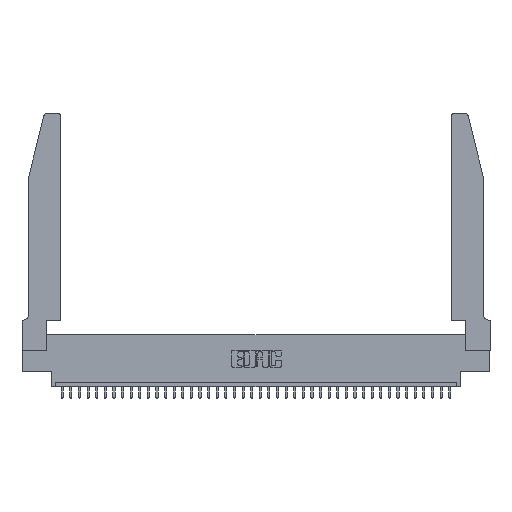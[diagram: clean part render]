
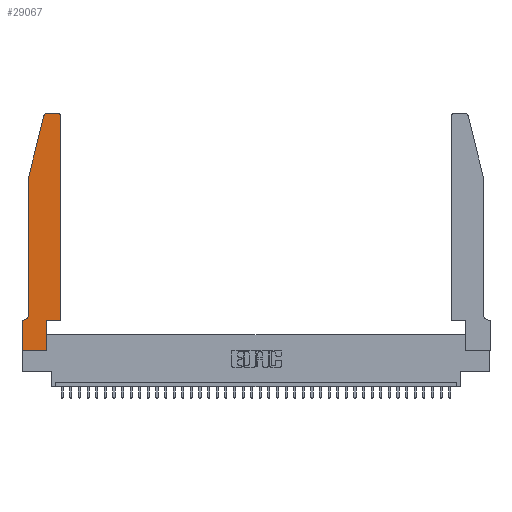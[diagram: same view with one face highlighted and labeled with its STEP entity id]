
A CAD part, top view. The second image highlights one B-rep face of the part: STEP entity #29067.
In plain terms, the highlighted planar face has unit normal (0, 0, 1).
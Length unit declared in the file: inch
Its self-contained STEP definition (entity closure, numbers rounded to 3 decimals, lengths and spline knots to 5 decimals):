
#1002 = CARTESIAN_POINT ( 'NONE',  ( 0.4505, 0.35, 0.37 ) ) ;
#1576 = VECTOR ( 'NONE', #4024, 39.37008 ) ;
#1795 = VECTOR ( 'NONE', #8593, 39.37008 ) ;
#1898 = CARTESIAN_POINT ( 'NONE',  ( 0.4205, 2.75, 0.37 ) ) ;
#2203 = VERTEX_POINT ( 'NONE', #10941 ) ;
#2248 = CARTESIAN_POINT ( 'NONE',  ( 0.25487, 2.72718, 0.37 ) ) ;
#2390 = LINE ( 'NONE', #22904, #25029 ) ;
#2543 = EDGE_CURVE ( 'NONE', #4899, #14342, #9378, .T. ) ;
#3140 = CARTESIAN_POINT ( 'NONE',  ( 0.2865, 0.35, 0.37 ) ) ;
#3373 = DIRECTION ( 'NONE',  ( 1., 0., 0. ) ) ;
#3374 = ORIENTED_EDGE ( 'NONE', *, *, #2543, .T. ) ;
#3980 = VERTEX_POINT ( 'NONE', #1002 ) ;
#4024 = DIRECTION ( 'NONE',  ( 0., -1., 0. ) ) ;
#4275 = CARTESIAN_POINT ( 'NONE',  ( 0., 0., 0.37 ) ) ;
#4356 = CARTESIAN_POINT ( 'NONE',  ( 0., 0.35, 0.37 ) ) ;
#4467 = CARTESIAN_POINT ( 'NONE',  ( 0.0755, 2., 0.37 ) ) ;
#4899 = VERTEX_POINT ( 'NONE', #8488 ) ;
#5185 = VECTOR ( 'NONE', #7511, 39.37008 ) ;
#5236 = DIRECTION ( 'NONE',  ( 0., -1., 0. ) ) ;
#5699 = EDGE_CURVE ( 'NONE', #17316, #4899, #7930, .T. ) ;
#5963 = VERTEX_POINT ( 'NONE', #2248 ) ;
#5990 = CIRCLE ( 'NONE', #24413, 0.03 ) ;
#6518 = ORIENTED_EDGE ( 'NONE', *, *, #33241, .T. ) ;
#7049 = CARTESIAN_POINT ( 'NONE',  ( 0.2605, 2.75, 0.37 ) ) ;
#7511 = DIRECTION ( 'NONE',  ( -0.239, -0.971, 0. ) ) ;
#7930 = LINE ( 'NONE', #4275, #25844 ) ;
#8007 = EDGE_CURVE ( 'NONE', #14342, #3980, #19101, .T. ) ;
#8199 = LINE ( 'NONE', #7049, #25663 ) ;
#8394 = CARTESIAN_POINT ( 'NONE',  ( 0., 0., 0.37 ) ) ;
#8488 = CARTESIAN_POINT ( 'NONE',  ( 0.2865, 0., 0.37 ) ) ;
#8521 = EDGE_CURVE ( 'NONE', #27605, #2203, #8199, .T. ) ;
#8593 = DIRECTION ( 'NONE',  ( -1., 0., 0. ) ) ;
#9063 = VECTOR ( 'NONE', #5236, 39.37008 ) ;
#9378 = LINE ( 'NONE', #3140, #13607 ) ;
#9404 = CARTESIAN_POINT ( 'NONE',  ( 0.4505, 2.72, 0.37 ) ) ;
#9760 = ORIENTED_EDGE ( 'NONE', *, *, #5699, .T. ) ;
#10782 = ORIENTED_EDGE ( 'NONE', *, *, #10862, .T. ) ;
#10862 = EDGE_CURVE ( 'NONE', #5963, #18989, #21683, .T. ) ;
#10941 = CARTESIAN_POINT ( 'NONE',  ( 0.284, 2.75, 0.37 ) ) ;
#12737 = EDGE_CURVE ( 'NONE', #27305, #31940, #38436, .T. ) ;
#13502 = AXIS2_PLACEMENT_3D ( 'NONE', #24848, #34447, #37445 ) ;
#13607 = VECTOR ( 'NONE', #33163, 39.37008 ) ;
#13802 = ORIENTED_EDGE ( 'NONE', *, *, #8521, .T. ) ;
#14062 = AXIS2_PLACEMENT_3D ( 'NONE', #14484, #27141, #3373 ) ;
#14342 = VERTEX_POINT ( 'NONE', #27661 ) ;
#14484 = CARTESIAN_POINT ( 'NONE',  ( 0., 0.35, 0.37 ) ) ;
#14936 = ORIENTED_EDGE ( 'NONE', *, *, #25347, .T. ) ;
#16009 = DIRECTION ( 'NONE',  ( 1., 0., 0. ) ) ;
#16510 = CARTESIAN_POINT ( 'NONE',  ( 0.0755, 0.35, 0.37 ) ) ;
#17316 = VERTEX_POINT ( 'NONE', #25467 ) ;
#17844 = LINE ( 'NONE', #16510, #1795 ) ;
#17965 = DIRECTION ( 'NONE',  ( 1., 0., 0. ) ) ;
#18018 = LINE ( 'NONE', #8394, #9063 ) ;
#18341 = ORIENTED_EDGE ( 'NONE', *, *, #29155, .T. ) ;
#18989 = VERTEX_POINT ( 'NONE', #28426 ) ;
#19101 = LINE ( 'NONE', #38603, #30384 ) ;
#19402 = ORIENTED_EDGE ( 'NONE', *, *, #21603, .T. ) ;
#19545 = EDGE_CURVE ( 'NONE', #2203, #5963, #34200, .T. ) ;
#21510 = VERTEX_POINT ( 'NONE', #9404 ) ;
#21603 = EDGE_CURVE ( 'NONE', #32172, #17316, #18018, .T. ) ;
#21683 = LINE ( 'NONE', #4467, #5185 ) ;
#22875 = DIRECTION ( 'NONE',  ( -1., 0., 0. ) ) ;
#22904 = CARTESIAN_POINT ( 'NONE',  ( 0.4505, 0.35, 0.37 ) ) ;
#23391 = DIRECTION ( 'NONE',  ( 0., 0., 1. ) ) ;
#23818 = AXIS2_PLACEMENT_3D ( 'NONE', #25109, #28149, #31546 ) ;
#24340 = PLANE ( 'NONE',  #14062 ) ;
#24413 = AXIS2_PLACEMENT_3D ( 'NONE', #32196, #23391, #32454 ) ;
#24729 = CARTESIAN_POINT ( 'NONE',  ( 0.0755, 0.42, 0.37 ) ) ;
#24848 = CARTESIAN_POINT ( 'NONE',  ( 0.0055, 0.42, 0.37 ) ) ;
#24993 = CARTESIAN_POINT ( 'NONE',  ( 0.0755, 2., 0.37 ) ) ;
#25029 = VECTOR ( 'NONE', #28830, 39.37008 ) ;
#25109 = CARTESIAN_POINT ( 'NONE',  ( 0.284, 2.72, 0.37 ) ) ;
#25347 = EDGE_CURVE ( 'NONE', #31940, #32172, #17844, .T. ) ;
#25467 = CARTESIAN_POINT ( 'NONE',  ( 0., 0., 0.37 ) ) ;
#25663 = VECTOR ( 'NONE', #22875, 39.37008 ) ;
#25844 = VECTOR ( 'NONE', #16009, 39.37008 ) ;
#27141 = DIRECTION ( 'NONE',  ( 0., 0., 1. ) ) ;
#27305 = VERTEX_POINT ( 'NONE', #24729 ) ;
#27511 = ORIENTED_EDGE ( 'NONE', *, *, #8007, .T. ) ;
#27605 = VERTEX_POINT ( 'NONE', #1898 ) ;
#27661 = CARTESIAN_POINT ( 'NONE',  ( 0.2865, 0.35, 0.37 ) ) ;
#28149 = DIRECTION ( 'NONE',  ( 0., 0., 1. ) ) ;
#28426 = CARTESIAN_POINT ( 'NONE',  ( 0.0755, 2., 0.37 ) ) ;
#28830 = DIRECTION ( 'NONE',  ( 0., 1., 0. ) ) ;
#29067 = ADVANCED_FACE ( 'NONE', ( #37762 ), #24340, .T. ) ;
#29155 = EDGE_CURVE ( 'NONE', #18989, #27305, #34622, .T. ) ;
#29888 = EDGE_CURVE ( 'NONE', #21510, #27605, #5990, .T. ) ;
#30384 = VECTOR ( 'NONE', #17965, 39.37008 ) ;
#31546 = DIRECTION ( 'NONE',  ( 1., 0., 0. ) ) ;
#31940 = VERTEX_POINT ( 'NONE', #38719 ) ;
#32172 = VERTEX_POINT ( 'NONE', #4356 ) ;
#32196 = CARTESIAN_POINT ( 'NONE',  ( 0.4205, 2.72, 0.37 ) ) ;
#32454 = DIRECTION ( 'NONE',  ( 1., 0., 0. ) ) ;
#32681 = EDGE_LOOP ( 'NONE', ( #13802, #37963, #10782, #18341, #37154, #14936, #19402, #9760, #3374, #27511, #6518, #37708 ) ) ;
#33163 = DIRECTION ( 'NONE',  ( 0., 1., 0. ) ) ;
#33241 = EDGE_CURVE ( 'NONE', #3980, #21510, #2390, .T. ) ;
#34200 = CIRCLE ( 'NONE', #23818, 0.03 ) ;
#34447 = DIRECTION ( 'NONE',  ( 0., 0., -1. ) ) ;
#34622 = LINE ( 'NONE', #24993, #1576 ) ;
#37154 = ORIENTED_EDGE ( 'NONE', *, *, #12737, .T. ) ;
#37445 = DIRECTION ( 'NONE',  ( -1., 0., 0. ) ) ;
#37708 = ORIENTED_EDGE ( 'NONE', *, *, #29888, .T. ) ;
#37762 = FACE_OUTER_BOUND ( 'NONE', #32681, .T. ) ;
#37963 = ORIENTED_EDGE ( 'NONE', *, *, #19545, .T. ) ;
#38436 = CIRCLE ( 'NONE', #13502, 0.07 ) ;
#38603 = CARTESIAN_POINT ( 'NONE',  ( 0.4505, 0.35, 0.37 ) ) ;
#38719 = CARTESIAN_POINT ( 'NONE',  ( 0.0055, 0.35, 0.37 ) ) ;
